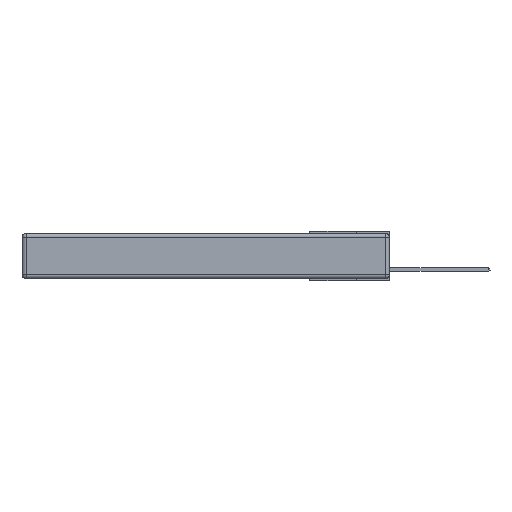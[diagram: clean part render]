
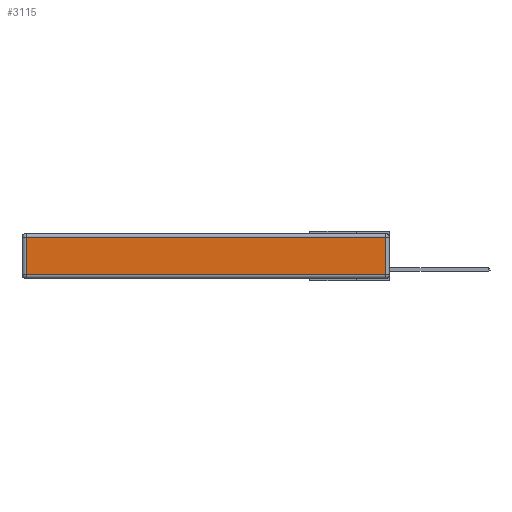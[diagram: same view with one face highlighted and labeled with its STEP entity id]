
A CAD part, left-side view. The second image highlights one B-rep face of the part: STEP entity #3115.
In plain terms, the highlighted planar face has unit normal (-1, 0, 0).
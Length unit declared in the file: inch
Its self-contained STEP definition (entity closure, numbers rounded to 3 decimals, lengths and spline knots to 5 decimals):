
#1448 = VERTEX_POINT ( 'NONE', #12912 ) ;
#1533 = AXIS2_PLACEMENT_3D ( 'NONE', #7800, #9821, #13289 ) ;
#1749 = ORIENTED_EDGE ( 'NONE', *, *, #20020, .T. ) ;
#2459 = VERTEX_POINT ( 'NONE', #13221 ) ;
#2662 = LINE ( 'NONE', #5649, #20611 ) ;
#3108 = CARTESIAN_POINT ( 'NONE',  ( 0., 0.03, -0.343 ) ) ;
#3115 = ADVANCED_FACE ( 'NONE', ( #3292 ), #6038, .T. ) ;
#3292 = FACE_OUTER_BOUND ( 'NONE', #9253, .T. ) ;
#4202 = CARTESIAN_POINT ( 'NONE',  ( 0., 2.72, -0.343 ) ) ;
#4752 = VECTOR ( 'NONE', #19469, 39.37008 ) ;
#5649 = CARTESIAN_POINT ( 'NONE',  ( 0., 2.75, -0.03 ) ) ;
#5879 = EDGE_CURVE ( 'NONE', #12120, #17725, #21720, .T. ) ;
#6038 = PLANE ( 'NONE',  #1533 ) ;
#7058 = ORIENTED_EDGE ( 'NONE', *, *, #19377, .T. ) ;
#7800 = CARTESIAN_POINT ( 'NONE',  ( 0., 0., -0.343 ) ) ;
#8753 = VECTOR ( 'NONE', #15837, 39.37008 ) ;
#9253 = EDGE_LOOP ( 'NONE', ( #1749, #7058, #21289, #16801 ) ) ;
#9821 = DIRECTION ( 'NONE',  ( -1., 0., 0. ) ) ;
#12120 = VERTEX_POINT ( 'NONE', #19569 ) ;
#12912 = CARTESIAN_POINT ( 'NONE',  ( 0., 0.03, -0.313 ) ) ;
#12982 = LINE ( 'NONE', #16078, #8753 ) ;
#13221 = CARTESIAN_POINT ( 'NONE',  ( 0., 0.03, -0.03 ) ) ;
#13289 = DIRECTION ( 'NONE',  ( 0., 0., 1. ) ) ;
#13348 = DIRECTION ( 'NONE',  ( 0., 0., -1. ) ) ;
#13595 = DIRECTION ( 'NONE',  ( 0., 1., 0. ) ) ;
#14003 = EDGE_CURVE ( 'NONE', #2459, #12120, #2662, .T. ) ;
#15837 = DIRECTION ( 'NONE',  ( 0., -1., 0. ) ) ;
#16078 = CARTESIAN_POINT ( 'NONE',  ( 0., 0., -0.313 ) ) ;
#16801 = ORIENTED_EDGE ( 'NONE', *, *, #5879, .T. ) ;
#17554 = LINE ( 'NONE', #3108, #4752 ) ;
#17725 = VERTEX_POINT ( 'NONE', #21871 ) ;
#19377 = EDGE_CURVE ( 'NONE', #1448, #2459, #17554, .T. ) ;
#19469 = DIRECTION ( 'NONE',  ( 0., 0., 1. ) ) ;
#19569 = CARTESIAN_POINT ( 'NONE',  ( 0., 2.72, -0.03 ) ) ;
#19966 = VECTOR ( 'NONE', #13348, 39.37008 ) ;
#20020 = EDGE_CURVE ( 'NONE', #17725, #1448, #12982, .T. ) ;
#20611 = VECTOR ( 'NONE', #13595, 39.37008 ) ;
#21289 = ORIENTED_EDGE ( 'NONE', *, *, #14003, .T. ) ;
#21720 = LINE ( 'NONE', #4202, #19966 ) ;
#21871 = CARTESIAN_POINT ( 'NONE',  ( 0., 2.72, -0.313 ) ) ;
